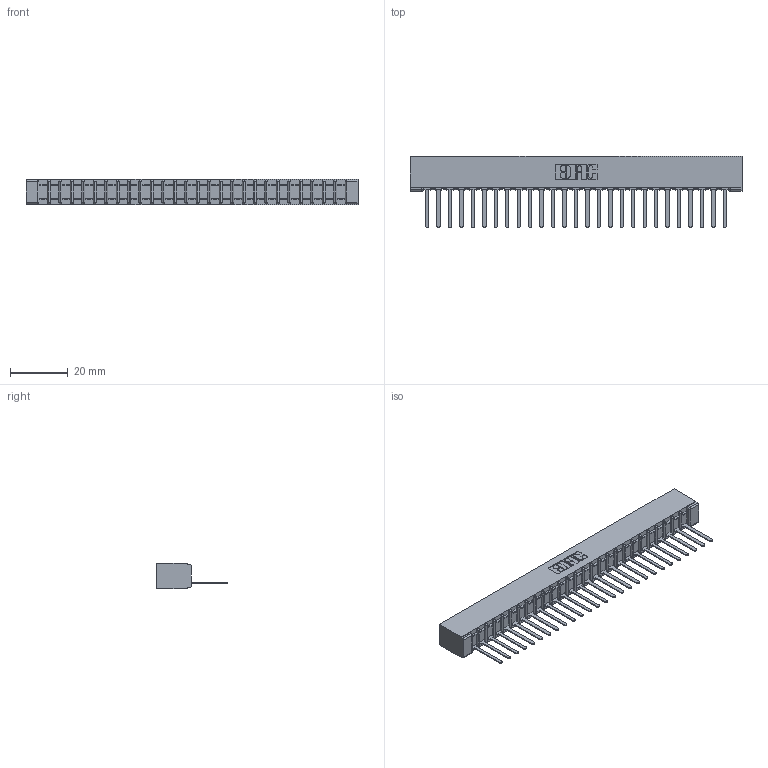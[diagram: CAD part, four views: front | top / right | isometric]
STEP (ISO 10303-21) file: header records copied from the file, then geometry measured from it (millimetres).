
FILE_DESCRIPTION (( 'STEP AP203' ), '1' );
FILE_NAME ('307-027-541-101.STEP', '2019-09-05T02:31:58', ( '' ), ( '' ), 'SwSTEP 2.0', 'SolidWorks 2016', '' );
FILE_SCHEMA (( 'CONFIG_CONTROL_DESIGN' ));
Length unit declared in the file: inch
Products named in the file (3): 307-027-541-101; 307-290-002_541; 307 Part_No Mounting Lugs
Assembly tree (28 placements, depth 2):
  307-027-541-101
    307 Part_No Mounting Lugs
    307-290-002_541  x27
Bounding box: 114.86 x 24.59 x 8.71 mm (x, y, z)
Volume: 7903.9 mm3; surface area: 15621.2 mm2
Topology: 28 solids, 28 shells, 2136 faces, 6563 edges, 4298 vertices
Faces by surface type: plane 1281, cylinder 799, sphere 56
Entity records: 25436 total; most frequent: CARTESIAN_POINT 4288, ORIENTED_EDGE 4278, DIRECTION 4171, EDGE_CURVE 2139, LINE 1633, VECTOR 1633, VERTEX_POINT 1386, AXIS2_PLACEMENT_3D 1269
